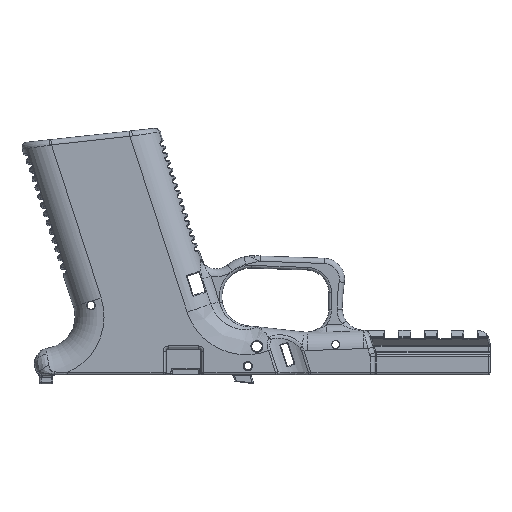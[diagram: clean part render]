
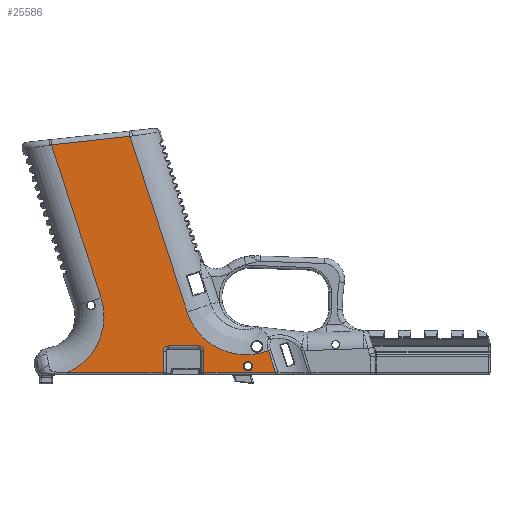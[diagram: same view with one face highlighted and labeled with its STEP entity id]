
A CAD part, front view. The second image highlights one B-rep face of the part: STEP entity #25586.
In plain terms, the highlighted planar face has unit normal (0, -1, 0).
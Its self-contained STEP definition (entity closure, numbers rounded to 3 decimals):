
#318=FACE_BOUND('',#7049,.T.);
#515=PLANE('',#28092);
#944=LINE('',#45964,#2269);
#990=LINE('',#50798,#2315);
#1524=LINE('',#59545,#2849);
#1525=LINE('',#59546,#2850);
#1526=LINE('',#59548,#2851);
#1527=LINE('',#59550,#2852);
#1528=LINE('',#59554,#2853);
#1529=LINE('',#59558,#2854);
#1530=LINE('',#59559,#2855);
#2269=VECTOR('',#30746,10.);
#2315=VECTOR('',#31282,10.);
#2849=VECTOR('',#33898,10.);
#2850=VECTOR('',#33899,10.);
#2851=VECTOR('',#33900,10.);
#2852=VECTOR('',#33901,10.);
#2853=VECTOR('',#33904,10.);
#2854=VECTOR('',#33907,10.);
#2855=VECTOR('',#33908,10.);
#5357=FACE_OUTER_BOUND('',#7048,.T.);
#7048=EDGE_LOOP('',(#21260,#21261,#21262,#21263,#21264,#21265,#21266,#21267,
#21268,#21269,#21270,#21271,#21272));
#7049=EDGE_LOOP('',(#21273));
#8097=CIRCLE('',#27213,23.01);
#8523=CIRCLE('',#28091,1.75);
#8524=CIRCLE('',#28093,2.);
#8525=CIRCLE('',#28094,2.);
#9689=B_SPLINE_CURVE_WITH_KNOTS('',3,(#59530,#59531,#59532,#59533,#59534,
#59535,#59536),.UNSPECIFIED.,.F.,.F.,(4,1,1,1,4),(0.,0.58,
1.74,2.9,3.82),.UNSPECIFIED.);
#10594=VERTEX_POINT('',#45961);
#10595=VERTEX_POINT('',#45963);
#10729=VERTEX_POINT('',#50795);
#10730=VERTEX_POINT('',#50797);
#10893=VERTEX_POINT('',#51836);
#11499=VERTEX_POINT('',#59513);
#11500=VERTEX_POINT('',#59540);
#11501=VERTEX_POINT('',#59544);
#11502=VERTEX_POINT('',#59547);
#11503=VERTEX_POINT('',#59549);
#11504=VERTEX_POINT('',#59551);
#11505=VERTEX_POINT('',#59553);
#11506=VERTEX_POINT('',#59555);
#11507=VERTEX_POINT('',#59557);
#13156=EDGE_CURVE('',#10594,#10595,#944,.T.);
#13476=EDGE_CURVE('',#10729,#10730,#990,.T.);
#13706=EDGE_CURVE('',#10893,#10729,#8097,.T.);
#14856=EDGE_CURVE('',#10595,#11499,#9689,.T.);
#14858=EDGE_CURVE('',#11500,#11500,#8523,.T.);
#14860=EDGE_CURVE('',#11499,#11501,#1524,.T.);
#14861=EDGE_CURVE('',#10730,#10594,#1525,.T.);
#14862=EDGE_CURVE('',#11502,#10893,#1526,.T.);
#14863=EDGE_CURVE('',#11503,#11502,#1527,.T.);
#14864=EDGE_CURVE('',#11504,#11503,#8524,.T.);
#14865=EDGE_CURVE('',#11505,#11504,#1528,.T.);
#14866=EDGE_CURVE('',#11506,#11505,#8525,.T.);
#14867=EDGE_CURVE('',#11507,#11506,#1529,.T.);
#14868=EDGE_CURVE('',#11501,#11507,#1530,.T.);
#21260=ORIENTED_EDGE('',*,*,#14860,.F.);
#21261=ORIENTED_EDGE('',*,*,#14856,.F.);
#21262=ORIENTED_EDGE('',*,*,#13156,.F.);
#21263=ORIENTED_EDGE('',*,*,#14861,.F.);
#21264=ORIENTED_EDGE('',*,*,#13476,.F.);
#21265=ORIENTED_EDGE('',*,*,#13706,.F.);
#21266=ORIENTED_EDGE('',*,*,#14862,.F.);
#21267=ORIENTED_EDGE('',*,*,#14863,.F.);
#21268=ORIENTED_EDGE('',*,*,#14864,.F.);
#21269=ORIENTED_EDGE('',*,*,#14865,.F.);
#21270=ORIENTED_EDGE('',*,*,#14866,.F.);
#21271=ORIENTED_EDGE('',*,*,#14867,.F.);
#21272=ORIENTED_EDGE('',*,*,#14868,.F.);
#21273=ORIENTED_EDGE('',*,*,#14858,.F.);
#25586=ADVANCED_FACE('',(#5357,#318),#515,.F.);
#27213=AXIS2_PLACEMENT_3D('',#51841,#31707,#31708);
#28091=AXIS2_PLACEMENT_3D('',#59541,#33893,#33894);
#28092=AXIS2_PLACEMENT_3D('',#59543,#33896,#33897);
#28093=AXIS2_PLACEMENT_3D('',#59552,#33902,#33903);
#28094=AXIS2_PLACEMENT_3D('',#59556,#33905,#33906);
#30746=DIRECTION('',(0.309,0.,-0.951));
#31282=DIRECTION('',(-0.309,0.,0.951));
#31707=DIRECTION('center_axis',(0.,-1.,0.));
#31708=DIRECTION('ref_axis',(0.864,0.,-0.504));
#33893=DIRECTION('center_axis',(0.,-1.,0.));
#33894=DIRECTION('ref_axis',(1.,0.,0.));
#33896=DIRECTION('center_axis',(0.,1.,0.));
#33897=DIRECTION('ref_axis',(1.,0.,0.));
#33898=DIRECTION('',(0.309,0.,-0.951));
#33899=DIRECTION('',(0.994,0.,0.108));
#33900=DIRECTION('',(-1.,0.,0.));
#33901=DIRECTION('',(0.,0.,-1.));
#33902=DIRECTION('center_axis',(0.,-1.,0.));
#33903=DIRECTION('ref_axis',(-0.707,0.,0.707));
#33904=DIRECTION('',(-1.,0.,0.));
#33905=DIRECTION('center_axis',(0.,-1.,0.));
#33906=DIRECTION('ref_axis',(0.707,0.,0.707));
#33907=DIRECTION('',(0.,0.,1.));
#33908=DIRECTION('',(-1.,0.,0.));
#45961=CARTESIAN_POINT('',(-43.553,-15.,50.503));
#45963=CARTESIAN_POINT('',(-21.903,-15.,-16.129));
#45964=CARTESIAN_POINT('',(-45.334,-15.,55.983));
#50795=CARTESIAN_POINT('',(-54.494,-15.,-10.792));
#50797=CARTESIAN_POINT('',(-73.358,-15.,47.266));
#50798=CARTESIAN_POINT('',(-64.362,-15.,19.58));
#51836=CARTESIAN_POINT('',(-67.193,-15.,-39.));
#51841=CARTESIAN_POINT('Origin',(-76.378,-15.,-17.902));
#59513=CARTESIAN_POINT('',(8.929,-15.,-30.782));
#59530=CARTESIAN_POINT('Ctrl Pts',(-21.903,-15.,-16.129));
#59531=CARTESIAN_POINT('Ctrl Pts',(-21.306,-15.,-17.967));
#59532=CARTESIAN_POINT('Ctrl Pts',(-18.824,-15.,-23.26));
#59533=CARTESIAN_POINT('Ctrl Pts',(-11.625,-15.,-30.143));
#59534=CARTESIAN_POINT('Ctrl Pts',(-0.894,-15.,-33.126));
#59535=CARTESIAN_POINT('Ctrl Pts',(6.068,-15.,-31.892));
#59536=CARTESIAN_POINT('Ctrl Pts',(8.928,-15.,-30.781));
#59540=CARTESIAN_POINT('',(-0.553,-15.,-36.614));
#59541=CARTESIAN_POINT('Origin',(1.197,-15.,-36.614));
#59543=CARTESIAN_POINT('Origin',(4.924,-15.,6.92));
#59544=CARTESIAN_POINT('',(11.599,-15.,-39.));
#59545=CARTESIAN_POINT('',(8.744,-15.,-30.214));
#59546=CARTESIAN_POINT('',(-41.628,-15.,50.713));
#59547=CARTESIAN_POINT('',(-31.,-15.,-39.));
#59548=CARTESIAN_POINT('',(48.962,-15.,-39.));
#59549=CARTESIAN_POINT('',(-31.,-15.,-31.));
#59550=CARTESIAN_POINT('',(-31.,-15.,-16.54));
#59551=CARTESIAN_POINT('',(-29.,-15.,-29.));
#59552=CARTESIAN_POINT('Origin',(-29.,-15.,-31.));
#59553=CARTESIAN_POINT('',(-17.5,-15.,-29.));
#59554=CARTESIAN_POINT('',(-12.538,-15.,-29.));
#59555=CARTESIAN_POINT('',(-15.5,-15.,-31.));
#59556=CARTESIAN_POINT('Origin',(-17.5,-15.,-31.));
#59557=CARTESIAN_POINT('',(-15.5,-15.,-39.));
#59558=CARTESIAN_POINT('',(-15.5,-15.,-11.54));
#59559=CARTESIAN_POINT('',(48.962,-15.,-39.));
